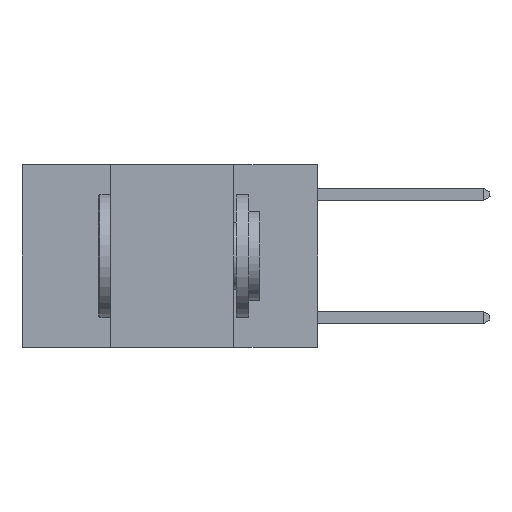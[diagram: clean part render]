
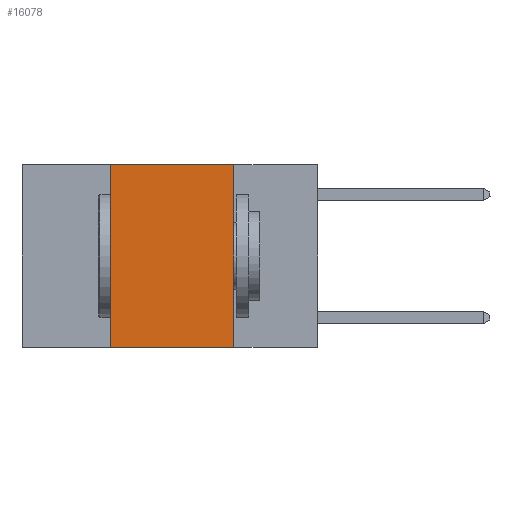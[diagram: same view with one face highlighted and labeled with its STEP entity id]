
A CAD part, left-side view. The second image highlights one B-rep face of the part: STEP entity #16078.
In plain terms, the highlighted planar face has unit normal (-1, 0, 0).
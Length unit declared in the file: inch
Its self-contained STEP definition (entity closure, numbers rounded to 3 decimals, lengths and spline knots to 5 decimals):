
#1606 = CARTESIAN_POINT ( 'NONE',  ( 0., 0.6, -0.37 ) ) ;
#1636 = VECTOR ( 'NONE', #16496, 39.37008 ) ;
#1782 = ORIENTED_EDGE ( 'NONE', *, *, #7703, .F. ) ;
#2244 = VECTOR ( 'NONE', #3859, 39.37008 ) ;
#2279 = CARTESIAN_POINT ( 'NONE',  ( 0., 0.17, 0. ) ) ;
#3334 = DIRECTION ( 'NONE',  ( 0., -1., 0. ) ) ;
#3859 = DIRECTION ( 'NONE',  ( 0., 0., 1. ) ) ;
#3942 = DIRECTION ( 'NONE',  ( 0., 0., -1. ) ) ;
#4521 = DIRECTION ( 'NONE',  ( 1., 0., 0. ) ) ;
#4615 = PLANE ( 'NONE',  #11425 ) ;
#4823 = CARTESIAN_POINT ( 'NONE',  ( 0., 0.17, -0.37 ) ) ;
#5000 = LINE ( 'NONE', #13916, #17771 ) ;
#5103 = EDGE_LOOP ( 'NONE', ( #6251, #1782, #15859, #5306 ) ) ;
#5306 = ORIENTED_EDGE ( 'NONE', *, *, #13754, .T. ) ;
#5317 = VERTEX_POINT ( 'NONE', #19164 ) ;
#5519 = CARTESIAN_POINT ( 'NONE',  ( 0., 0.42, 0. ) ) ;
#5538 = EDGE_CURVE ( 'NONE', #5317, #6182, #6804, .T. ) ;
#5945 = VERTEX_POINT ( 'NONE', #8062 ) ;
#6182 = VERTEX_POINT ( 'NONE', #17933 ) ;
#6251 = ORIENTED_EDGE ( 'NONE', *, *, #18491, .F. ) ;
#6804 = LINE ( 'NONE', #5519, #2244 ) ;
#7703 = EDGE_CURVE ( 'NONE', #6182, #5945, #5000, .T. ) ;
#8062 = CARTESIAN_POINT ( 'NONE',  ( 0., 0.17, 0. ) ) ;
#10358 = LINE ( 'NONE', #1606, #1636 ) ;
#11311 = LINE ( 'NONE', #2279, #16169 ) ;
#11425 = AXIS2_PLACEMENT_3D ( 'NONE', #11978, #4521, #13528 ) ;
#11978 = CARTESIAN_POINT ( 'NONE',  ( 0., 0.6, 0. ) ) ;
#13528 = DIRECTION ( 'NONE',  ( 0., 0., -1. ) ) ;
#13754 = EDGE_CURVE ( 'NONE', #5317, #18886, #10358, .T. ) ;
#13916 = CARTESIAN_POINT ( 'NONE',  ( 0., 0.6, 0. ) ) ;
#14895 = FACE_OUTER_BOUND ( 'NONE', #5103, .T. ) ;
#15859 = ORIENTED_EDGE ( 'NONE', *, *, #5538, .F. ) ;
#16078 = ADVANCED_FACE ( 'NONE', ( #14895 ), #4615, .F. ) ;
#16169 = VECTOR ( 'NONE', #3942, 39.37008 ) ;
#16496 = DIRECTION ( 'NONE',  ( 0., -1., 0. ) ) ;
#17771 = VECTOR ( 'NONE', #3334, 39.37008 ) ;
#17933 = CARTESIAN_POINT ( 'NONE',  ( 0., 0.42, 0. ) ) ;
#18491 = EDGE_CURVE ( 'NONE', #5945, #18886, #11311, .T. ) ;
#18886 = VERTEX_POINT ( 'NONE', #4823 ) ;
#19164 = CARTESIAN_POINT ( 'NONE',  ( 0., 0.42, -0.37 ) ) ;
